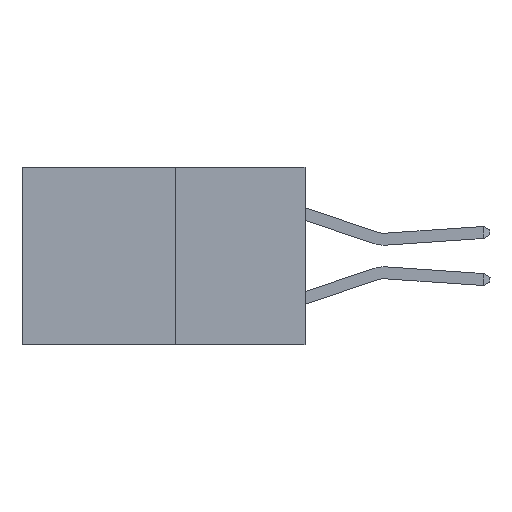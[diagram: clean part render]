
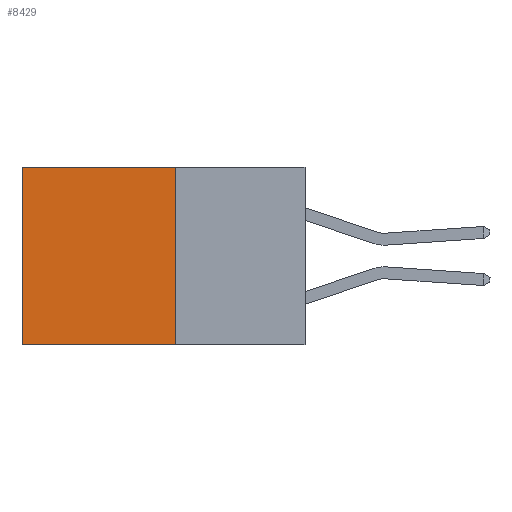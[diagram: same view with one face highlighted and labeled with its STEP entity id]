
A CAD part, left-side view. The second image highlights one B-rep face of the part: STEP entity #8429.
In plain terms, the highlighted planar face has unit normal (-1, 0, 0).
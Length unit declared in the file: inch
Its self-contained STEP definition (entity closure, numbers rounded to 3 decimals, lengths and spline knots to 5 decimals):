
#464 = ORIENTED_EDGE ( 'NONE', *, *, #22299, .T. ) ;
#536 = FACE_OUTER_BOUND ( 'NONE', #19782, .T. ) ;
#610 = VERTEX_POINT ( 'NONE', #22922 ) ;
#3021 = CARTESIAN_POINT ( 'NONE',  ( 0.277, 0.27, -0.37 ) ) ;
#3698 = EDGE_CURVE ( 'NONE', #610, #20807, #29015, .T. ) ;
#4523 = CARTESIAN_POINT ( 'NONE',  ( 0.277, 0.27, -0.37 ) ) ;
#4794 = CARTESIAN_POINT ( 'NONE',  ( 0.277, 0.27, -0.37 ) ) ;
#5057 = DIRECTION ( 'NONE',  ( 0., 0., -1. ) ) ;
#5316 = LINE ( 'NONE', #10077, #18711 ) ;
#5513 = CARTESIAN_POINT ( 'NONE',  ( 0.277, 0.59, -0.37 ) ) ;
#5641 = DIRECTION ( 'NONE',  ( 0., 0., -1. ) ) ;
#5922 = VERTEX_POINT ( 'NONE', #13055 ) ;
#5956 = ORIENTED_EDGE ( 'NONE', *, *, #26934, .F. ) ;
#7376 = DIRECTION ( 'NONE',  ( 0., 1., 0. ) ) ;
#7581 = VERTEX_POINT ( 'NONE', #4523 ) ;
#7863 = VECTOR ( 'NONE', #5057, 39.37008 ) ;
#8429 = ADVANCED_FACE ( 'NONE', ( #536 ), #10950, .F. ) ;
#9160 = EDGE_CURVE ( 'NONE', #7581, #20807, #26698, .T. ) ;
#10077 = CARTESIAN_POINT ( 'NONE',  ( 0.277, 0.27, 0. ) ) ;
#10950 = PLANE ( 'NONE',  #33325 ) ;
#13055 = CARTESIAN_POINT ( 'NONE',  ( 0.277, 0.27, 0. ) ) ;
#13701 = VECTOR ( 'NONE', #28732, 39.37008 ) ;
#14527 = LINE ( 'NONE', #4794, #13701 ) ;
#15847 = ORIENTED_EDGE ( 'NONE', *, *, #9160, .F. ) ;
#15949 = VECTOR ( 'NONE', #24352, 39.37008 ) ;
#18711 = VECTOR ( 'NONE', #7376, 39.37008 ) ;
#18984 = CARTESIAN_POINT ( 'NONE',  ( 0.277, 0.27, -0.37 ) ) ;
#19782 = EDGE_LOOP ( 'NONE', ( #32172, #15847, #5956, #464 ) ) ;
#20807 = VERTEX_POINT ( 'NONE', #31034 ) ;
#21630 = DIRECTION ( 'NONE',  ( 1., 0., 0. ) ) ;
#22299 = EDGE_CURVE ( 'NONE', #5922, #610, #5316, .T. ) ;
#22922 = CARTESIAN_POINT ( 'NONE',  ( 0.277, 0.59, 0. ) ) ;
#24352 = DIRECTION ( 'NONE',  ( 0., 1., 0. ) ) ;
#26698 = LINE ( 'NONE', #3021, #15949 ) ;
#26934 = EDGE_CURVE ( 'NONE', #5922, #7581, #14527, .T. ) ;
#28732 = DIRECTION ( 'NONE',  ( 0., 0., -1. ) ) ;
#29015 = LINE ( 'NONE', #5513, #7863 ) ;
#31034 = CARTESIAN_POINT ( 'NONE',  ( 0.277, 0.59, -0.37 ) ) ;
#32172 = ORIENTED_EDGE ( 'NONE', *, *, #3698, .T. ) ;
#33325 = AXIS2_PLACEMENT_3D ( 'NONE', #18984, #21630, #5641 ) ;
